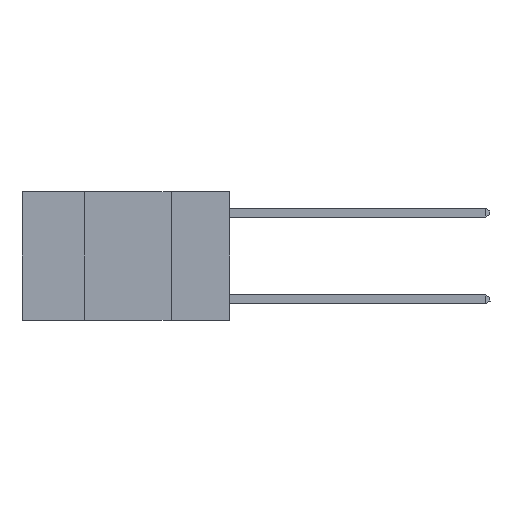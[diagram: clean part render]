
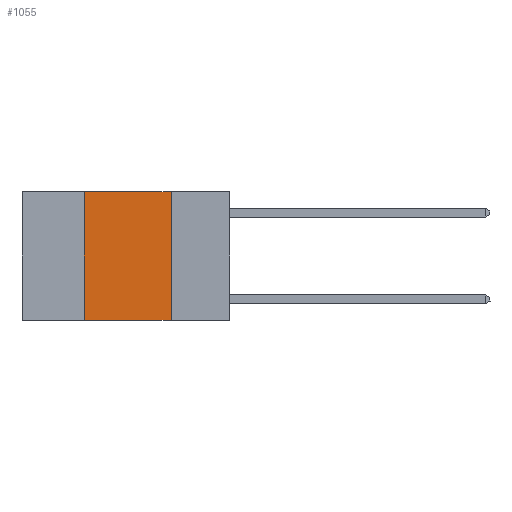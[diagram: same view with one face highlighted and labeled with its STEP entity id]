
A CAD part, left-side view. The second image highlights one B-rep face of the part: STEP entity #1055.
In plain terms, the highlighted planar face has unit normal (-1, 0, 0).
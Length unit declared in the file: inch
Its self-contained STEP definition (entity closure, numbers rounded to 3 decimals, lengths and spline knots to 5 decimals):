
#349 = CARTESIAN_POINT ( 'NONE',  ( 0., 0.6, -0.37 ) ) ;
#536 = AXIS2_PLACEMENT_3D ( 'NONE', #6369, #2865, #11102 ) ;
#897 = DIRECTION ( 'NONE',  ( 0., -1., 0. ) ) ;
#1055 = ADVANCED_FACE ( 'NONE', ( #7761 ), #9942, .F. ) ;
#1162 = VERTEX_POINT ( 'NONE', #14983 ) ;
#1432 = VERTEX_POINT ( 'NONE', #1900 ) ;
#1451 = CARTESIAN_POINT ( 'NONE',  ( 0., 0.42, 0. ) ) ;
#1900 = CARTESIAN_POINT ( 'NONE',  ( 0., 0.42, -0.37 ) ) ;
#2591 = CARTESIAN_POINT ( 'NONE',  ( 0., 0.17, -0.37 ) ) ;
#2678 = VECTOR ( 'NONE', #6364, 39.37008 ) ;
#2865 = DIRECTION ( 'NONE',  ( 1., 0., 0. ) ) ;
#3842 = CARTESIAN_POINT ( 'NONE',  ( 0., 0.42, 0. ) ) ;
#5860 = VECTOR ( 'NONE', #10191, 39.37008 ) ;
#6247 = EDGE_CURVE ( 'NONE', #7979, #1162, #12450, .T. ) ;
#6248 = VECTOR ( 'NONE', #897, 39.37008 ) ;
#6364 = DIRECTION ( 'NONE',  ( 0., -1., 0. ) ) ;
#6369 = CARTESIAN_POINT ( 'NONE',  ( 0., 0.6, 0. ) ) ;
#7443 = DIRECTION ( 'NONE',  ( 0., 0., 1. ) ) ;
#7761 = FACE_OUTER_BOUND ( 'NONE', #8553, .T. ) ;
#7805 = CARTESIAN_POINT ( 'NONE',  ( 0., 0.17, 0. ) ) ;
#7979 = VERTEX_POINT ( 'NONE', #1451 ) ;
#8080 = EDGE_CURVE ( 'NONE', #1432, #8595, #8946, .T. ) ;
#8233 = ORIENTED_EDGE ( 'NONE', *, *, #15095, .F. ) ;
#8287 = VECTOR ( 'NONE', #7443, 39.37008 ) ;
#8509 = ORIENTED_EDGE ( 'NONE', *, *, #6247, .F. ) ;
#8553 = EDGE_LOOP ( 'NONE', ( #8233, #8509, #9006, #9580 ) ) ;
#8595 = VERTEX_POINT ( 'NONE', #2591 ) ;
#8946 = LINE ( 'NONE', #349, #2678 ) ;
#9006 = ORIENTED_EDGE ( 'NONE', *, *, #13537, .F. ) ;
#9580 = ORIENTED_EDGE ( 'NONE', *, *, #8080, .T. ) ;
#9942 = PLANE ( 'NONE',  #536 ) ;
#10191 = DIRECTION ( 'NONE',  ( 0., 0., -1. ) ) ;
#11102 = DIRECTION ( 'NONE',  ( 0., 0., -1. ) ) ;
#11353 = LINE ( 'NONE', #7805, #5860 ) ;
#11382 = LINE ( 'NONE', #3842, #8287 ) ;
#11531 = CARTESIAN_POINT ( 'NONE',  ( 0., 0.6, 0. ) ) ;
#12450 = LINE ( 'NONE', #11531, #6248 ) ;
#13537 = EDGE_CURVE ( 'NONE', #1432, #7979, #11382, .T. ) ;
#14983 = CARTESIAN_POINT ( 'NONE',  ( 0., 0.17, 0. ) ) ;
#15095 = EDGE_CURVE ( 'NONE', #1162, #8595, #11353, .T. ) ;
